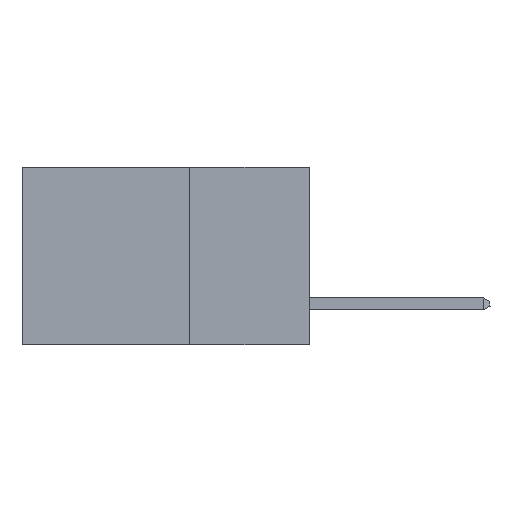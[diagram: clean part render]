
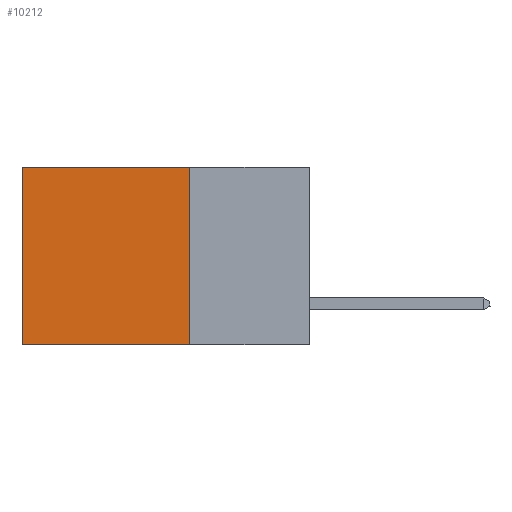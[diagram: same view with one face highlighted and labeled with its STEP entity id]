
A CAD part, left-side view. The second image highlights one B-rep face of the part: STEP entity #10212.
In plain terms, the highlighted planar face has unit normal (-1, 0, 0).
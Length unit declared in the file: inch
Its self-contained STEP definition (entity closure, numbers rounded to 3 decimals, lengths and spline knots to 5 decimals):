
#372 = EDGE_CURVE ( 'NONE', #17983, #945, #6152, .T. ) ;
#668 = VECTOR ( 'NONE', #7652, 39.37008 ) ;
#932 = VECTOR ( 'NONE', #15994, 39.37008 ) ;
#945 = VERTEX_POINT ( 'NONE', #15323 ) ;
#1329 = ORIENTED_EDGE ( 'NONE', *, *, #22747, .T. ) ;
#2033 = LINE ( 'NONE', #24607, #15217 ) ;
#2287 = VERTEX_POINT ( 'NONE', #4632 ) ;
#3773 = CARTESIAN_POINT ( 'NONE',  ( 0.2875, 0.25, 0. ) ) ;
#4223 = DIRECTION ( 'NONE',  ( 0., 0., -1. ) ) ;
#4296 = CARTESIAN_POINT ( 'NONE',  ( 0.2875, 0.25, -0.37 ) ) ;
#4448 = LINE ( 'NONE', #9648, #932 ) ;
#4632 = CARTESIAN_POINT ( 'NONE',  ( 0.2875, 0.25, -0.37 ) ) ;
#5114 = AXIS2_PLACEMENT_3D ( 'NONE', #3773, #18359, #4223 ) ;
#6152 = LINE ( 'NONE', #15579, #668 ) ;
#6815 = ORIENTED_EDGE ( 'NONE', *, *, #26608, .F. ) ;
#7652 = DIRECTION ( 'NONE',  ( 0., 1., 0. ) ) ;
#8284 = DIRECTION ( 'NONE',  ( 0., 0., -1. ) ) ;
#8471 = VECTOR ( 'NONE', #18686, 39.37008 ) ;
#9648 = CARTESIAN_POINT ( 'NONE',  ( 0.2875, 0.6, 0. ) ) ;
#10212 = ADVANCED_FACE ( 'NONE', ( #10306 ), #21835, .F. ) ;
#10306 = FACE_OUTER_BOUND ( 'NONE', #18857, .T. ) ;
#12396 = VERTEX_POINT ( 'NONE', #21908 ) ;
#15217 = VECTOR ( 'NONE', #8284, 39.37008 ) ;
#15323 = CARTESIAN_POINT ( 'NONE',  ( 0.2875, 0.6, 0. ) ) ;
#15579 = CARTESIAN_POINT ( 'NONE',  ( 0.2875, 0.25, 0. ) ) ;
#15994 = DIRECTION ( 'NONE',  ( 0., 0., -1. ) ) ;
#17983 = VERTEX_POINT ( 'NONE', #20858 ) ;
#18359 = DIRECTION ( 'NONE',  ( 1., 0., 0. ) ) ;
#18686 = DIRECTION ( 'NONE',  ( 0., 1., 0. ) ) ;
#18857 = EDGE_LOOP ( 'NONE', ( #1329, #22866, #6815, #22521 ) ) ;
#20555 = EDGE_CURVE ( 'NONE', #2287, #12396, #26425, .T. ) ;
#20858 = CARTESIAN_POINT ( 'NONE',  ( 0.2875, 0.25, 0. ) ) ;
#21835 = PLANE ( 'NONE',  #5114 ) ;
#21908 = CARTESIAN_POINT ( 'NONE',  ( 0.2875, 0.6, -0.37 ) ) ;
#22521 = ORIENTED_EDGE ( 'NONE', *, *, #372, .T. ) ;
#22747 = EDGE_CURVE ( 'NONE', #945, #12396, #4448, .T. ) ;
#22866 = ORIENTED_EDGE ( 'NONE', *, *, #20555, .F. ) ;
#24607 = CARTESIAN_POINT ( 'NONE',  ( 0.2875, 0.25, 0. ) ) ;
#26425 = LINE ( 'NONE', #4296, #8471 ) ;
#26608 = EDGE_CURVE ( 'NONE', #17983, #2287, #2033, .T. ) ;
